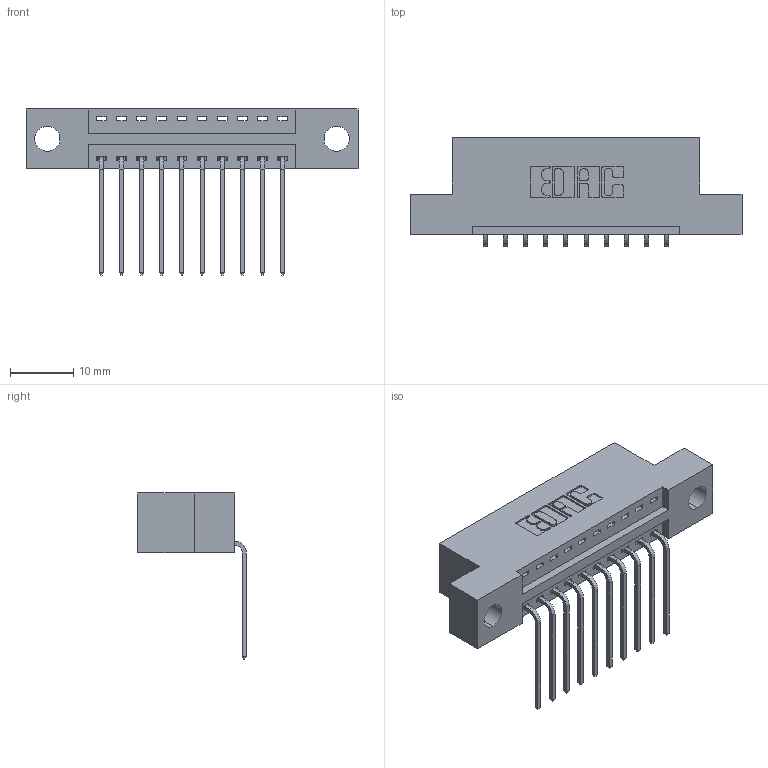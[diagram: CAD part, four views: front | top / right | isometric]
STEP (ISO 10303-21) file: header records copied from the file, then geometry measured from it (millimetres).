
FILE_DESCRIPTION (( 'STEP AP203' ), '1' );
FILE_NAME ('346-010-559-104.STEP', '2022-05-05T00:25:07', ( '' ), ( '' ), 'SwSTEP 2.0', 'SolidWorks 2020', '' );
FILE_SCHEMA (( 'CONFIG_CONTROL_DESIGN' ));
Length unit declared in the file: inch
Products named in the file (3): 346 Part_Flush Mounting Lugs - 0.156 Dia-TH; 345-292-001_558 559 Tail - 1; 346-010-559-104
Assembly tree (11 placements, depth 2):
  346-010-559-104
    346 Part_Flush Mounting Lugs - 0.156 Dia-TH
    345-292-001_558 559 Tail - 1  x10
Bounding box: 52.32 x 17.08 x 26.16 mm (x, y, z)
Volume: 4715.5 mm3; surface area: 5584.4 mm2
Topology: 11 solids, 11 shells, 736 faces, 2185 edges, 1442 vertices
Faces by surface type: plane 510, cylinder 226
Entity records: 11017 total; most frequent: CARTESIAN_POINT 1908, ORIENTED_EDGE 1850, DIRECTION 1721, EDGE_CURVE 925, LINE 753, VECTOR 753, VERTEX_POINT 614, AXIS2_PLACEMENT_3D 484
